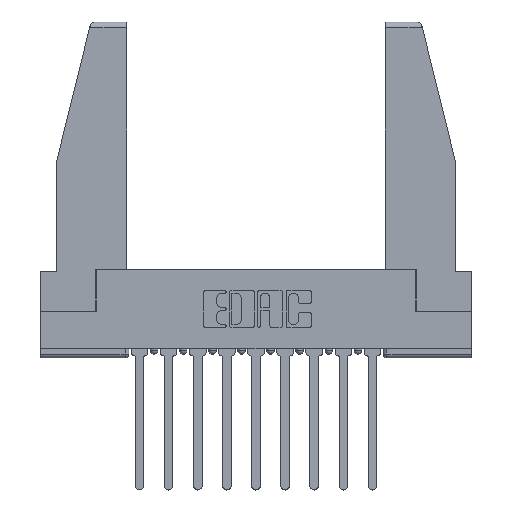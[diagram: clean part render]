
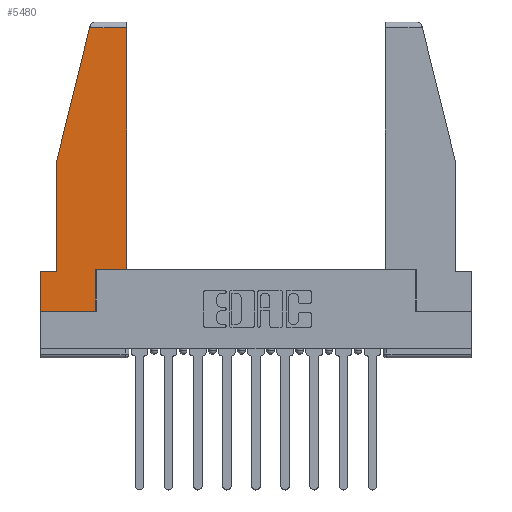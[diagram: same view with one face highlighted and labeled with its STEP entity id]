
A CAD part, top view. The second image highlights one B-rep face of the part: STEP entity #5480.
In plain terms, the highlighted planar face has unit normal (0, 0, 1).
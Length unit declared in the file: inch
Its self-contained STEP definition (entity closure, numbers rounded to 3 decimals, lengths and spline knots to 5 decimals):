
#210 = CARTESIAN_POINT ( 'NONE',  ( 0.297, 0., 0. ) ) ;
#404 = DIRECTION ( 'NONE',  ( -1., 0., 0. ) ) ;
#547 = EDGE_CURVE ( 'NONE', #13978, #3970, #11636, .T. ) ;
#682 = FACE_OUTER_BOUND ( 'NONE', #9750, .T. ) ;
#780 = DIRECTION ( 'NONE',  ( 0., 1., 0. ) ) ;
#1251 = VECTOR ( 'NONE', #12483, 39.37008 ) ;
#1644 = VERTEX_POINT ( 'NONE', #13926 ) ;
#1653 = VERTEX_POINT ( 'NONE', #3071 ) ;
#2295 = CARTESIAN_POINT ( 'NONE',  ( 0., 0., 0. ) ) ;
#2924 = ORIENTED_EDGE ( 'NONE', *, *, #547, .T. ) ;
#3040 = VECTOR ( 'NONE', #404, 39.37008 ) ;
#3071 = CARTESIAN_POINT ( 'NONE',  ( 0., 0.21, 0. ) ) ;
#3072 = VECTOR ( 'NONE', #13039, 39.37008 ) ;
#3189 = ORIENTED_EDGE ( 'NONE', *, *, #4246, .T. ) ;
#3606 = VERTEX_POINT ( 'NONE', #10894 ) ;
#3658 = LINE ( 'NONE', #12376, #9814 ) ;
#3970 = VERTEX_POINT ( 'NONE', #4450 ) ;
#4035 = ORIENTED_EDGE ( 'NONE', *, *, #9671, .T. ) ;
#4115 = ORIENTED_EDGE ( 'NONE', *, *, #11545, .T. ) ;
#4246 = EDGE_CURVE ( 'NONE', #7417, #3606, #12124, .T. ) ;
#4273 = AXIS2_PLACEMENT_3D ( 'NONE', #8331, #12689, #6041 ) ;
#4348 = EDGE_CURVE ( 'NONE', #14069, #1653, #5682, .T. ) ;
#4450 = CARTESIAN_POINT ( 'NONE',  ( 0.2636, 1.52, 0. ) ) ;
#5216 = ORIENTED_EDGE ( 'NONE', *, *, #9798, .T. ) ;
#5480 = ADVANCED_FACE ( 'NONE', ( #682 ), #13639, .T. ) ;
#5682 = LINE ( 'NONE', #6745, #3072 ) ;
#5809 = LINE ( 'NONE', #6822, #11867 ) ;
#6041 = DIRECTION ( 'NONE',  ( 1., 0., 0. ) ) ;
#6208 = DIRECTION ( 'NONE',  ( -0.239, -0.971, 0. ) ) ;
#6745 = CARTESIAN_POINT ( 'NONE',  ( 0., 0.21, 0. ) ) ;
#6760 = CARTESIAN_POINT ( 'NONE',  ( 0.461, 1.52, 0. ) ) ;
#6785 = VECTOR ( 'NONE', #6208, 39.37008 ) ;
#6822 = CARTESIAN_POINT ( 'NONE',  ( 0.297, 0.223, 0. ) ) ;
#6959 = DIRECTION ( 'NONE',  ( 0., -1., 0. ) ) ;
#7417 = VERTEX_POINT ( 'NONE', #13189 ) ;
#7539 = VECTOR ( 'NONE', #780, 39.37008 ) ;
#7707 = VERTEX_POINT ( 'NONE', #10893 ) ;
#8033 = DIRECTION ( 'NONE',  ( 0., -1., 0. ) ) ;
#8168 = ORIENTED_EDGE ( 'NONE', *, *, #12861, .T. ) ;
#8203 = VECTOR ( 'NONE', #8033, 39.37008 ) ;
#8331 = CARTESIAN_POINT ( 'NONE',  ( 0., 0., 0. ) ) ;
#8569 = LINE ( 'NONE', #10865, #7539 ) ;
#8912 = ORIENTED_EDGE ( 'NONE', *, *, #4348, .T. ) ;
#9059 = LINE ( 'NONE', #210, #1251 ) ;
#9103 = LINE ( 'NONE', #10270, #8203 ) ;
#9671 = EDGE_CURVE ( 'NONE', #3606, #10110, #9059, .T. ) ;
#9750 = EDGE_LOOP ( 'NONE', ( #12502, #2924, #5216, #8168, #8912, #10491, #3189, #4035, #4115 ) ) ;
#9798 = EDGE_CURVE ( 'NONE', #3970, #1644, #13808, .T. ) ;
#9814 = VECTOR ( 'NONE', #6959, 39.37008 ) ;
#10110 = VERTEX_POINT ( 'NONE', #10285 ) ;
#10270 = CARTESIAN_POINT ( 'NONE',  ( 0., 0.21, 0. ) ) ;
#10285 = CARTESIAN_POINT ( 'NONE',  ( 0.297, 0.223, 0. ) ) ;
#10491 = ORIENTED_EDGE ( 'NONE', *, *, #14186, .T. ) ;
#10865 = CARTESIAN_POINT ( 'NONE',  ( 0.461, 0.223, 0. ) ) ;
#10893 = CARTESIAN_POINT ( 'NONE',  ( 0.461, 0.223, 0. ) ) ;
#10894 = CARTESIAN_POINT ( 'NONE',  ( 0.297, 0., 0. ) ) ;
#11066 = DIRECTION ( 'NONE',  ( 1., 0., 0. ) ) ;
#11545 = EDGE_CURVE ( 'NONE', #10110, #7707, #5809, .T. ) ;
#11636 = LINE ( 'NONE', #12555, #3040 ) ;
#11867 = VECTOR ( 'NONE', #12238, 39.37008 ) ;
#11999 = EDGE_CURVE ( 'NONE', #7707, #13978, #8569, .T. ) ;
#12124 = LINE ( 'NONE', #2295, #13240 ) ;
#12238 = DIRECTION ( 'NONE',  ( 1., 0., 0. ) ) ;
#12376 = CARTESIAN_POINT ( 'NONE',  ( 0.086, 0.8, 0. ) ) ;
#12483 = DIRECTION ( 'NONE',  ( 0., 1., 0. ) ) ;
#12502 = ORIENTED_EDGE ( 'NONE', *, *, #11999, .T. ) ;
#12555 = CARTESIAN_POINT ( 'NONE',  ( 0., 1.52, 0. ) ) ;
#12689 = DIRECTION ( 'NONE',  ( 0., 0., 1. ) ) ;
#12859 = CARTESIAN_POINT ( 'NONE',  ( 0.271, 1.55, 0. ) ) ;
#12861 = EDGE_CURVE ( 'NONE', #1644, #14069, #3658, .T. ) ;
#13039 = DIRECTION ( 'NONE',  ( -1., 0., 0. ) ) ;
#13120 = CARTESIAN_POINT ( 'NONE',  ( 0.086, 0.21, 0. ) ) ;
#13189 = CARTESIAN_POINT ( 'NONE',  ( 0., 0., 0. ) ) ;
#13240 = VECTOR ( 'NONE', #11066, 39.37008 ) ;
#13639 = PLANE ( 'NONE',  #4273 ) ;
#13808 = LINE ( 'NONE', #12859, #6785 ) ;
#13926 = CARTESIAN_POINT ( 'NONE',  ( 0.086, 0.8, 0. ) ) ;
#13978 = VERTEX_POINT ( 'NONE', #6760 ) ;
#14069 = VERTEX_POINT ( 'NONE', #13120 ) ;
#14186 = EDGE_CURVE ( 'NONE', #1653, #7417, #9103, .T. ) ;
